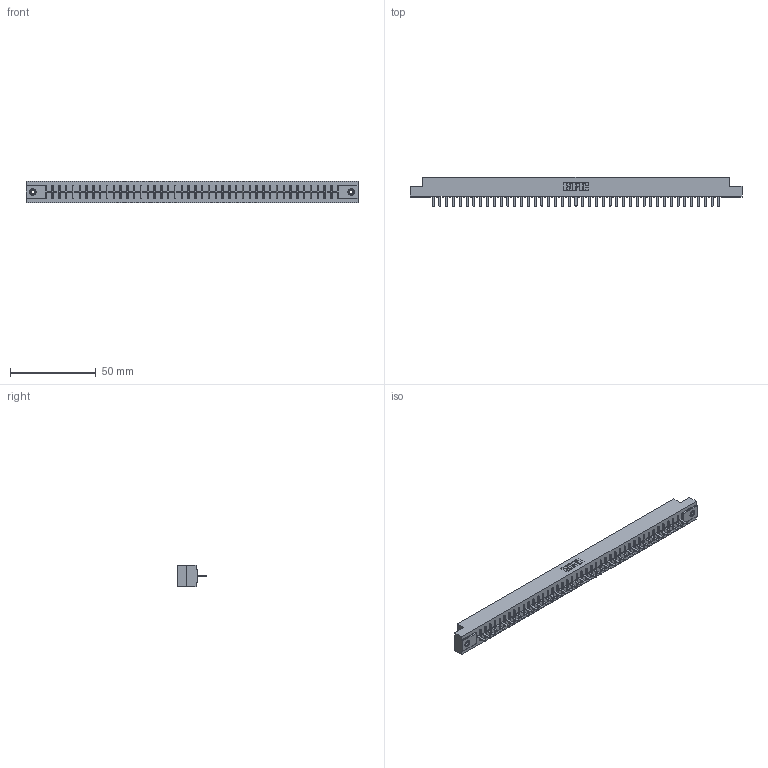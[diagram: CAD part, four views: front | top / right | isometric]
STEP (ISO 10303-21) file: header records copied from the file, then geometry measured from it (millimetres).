
FILE_DESCRIPTION (( 'STEP AP203' ), '1' );
FILE_NAME ('306-043-520-108.STEP', '2019-09-12T01:04:39', ( '' ), ( '' ), 'SwSTEP 2.0', 'SolidWorks 2016', '' );
FILE_SCHEMA (( 'CONFIG_CONTROL_DESIGN' ));
Length unit declared in the file: inch
Products named in the file (4): 306 Part_.156 Dia; 306-290-001_120; 345-250-001_345-250-003-102; 306-043-520-108
Assembly tree (46 placements, depth 2):
  306-043-520-108
    306 Part_.156 Dia
    306-290-001_120  x43
    345-250-001_345-250-003-102  x2
Bounding box: 193.4 x 17.12 x 12.7 mm (x, y, z)
Volume: 21396.8 mm3; surface area: 22016.4 mm2
Topology: 46 solids, 46 shells, 3186 faces, 8923 edges, 5710 vertices
Faces by surface type: plane 2121, cylinder 877, sphere 172, cone 12, torus 4
Entity records: 41111 total; most frequent: CARTESIAN_POINT 6883, ORIENTED_EDGE 6818, DIRECTION 6795, EDGE_CURVE 3409, VECTOR 2667, LINE 2667, VERTEX_POINT 2152, AXIS2_PLACEMENT_3D 2064
